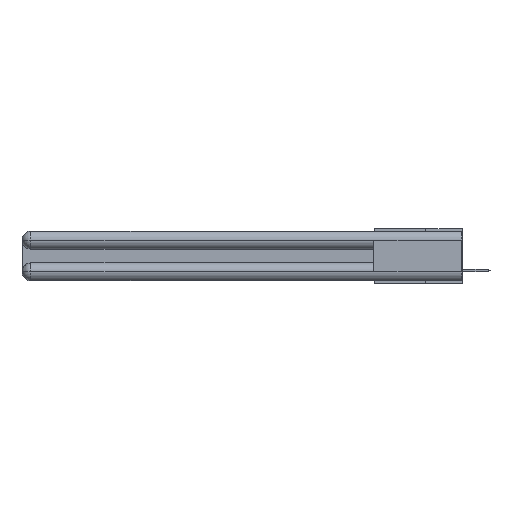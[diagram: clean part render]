
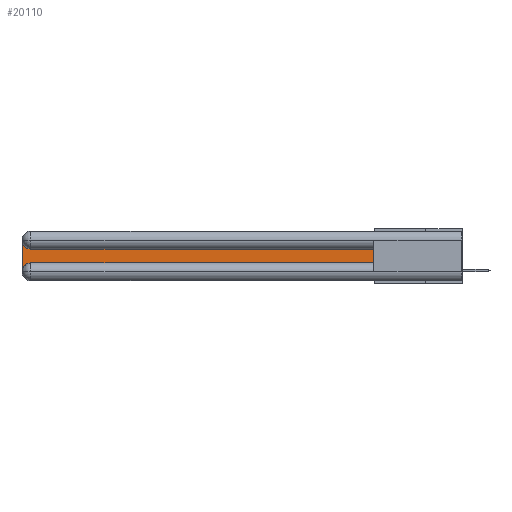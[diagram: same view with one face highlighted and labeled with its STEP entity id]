
A CAD part, left-side view. The second image highlights one B-rep face of the part: STEP entity #20110.
In plain terms, the highlighted planar face has unit normal (-1, 0, 0).
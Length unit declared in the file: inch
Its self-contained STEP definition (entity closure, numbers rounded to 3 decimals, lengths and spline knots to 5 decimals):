
#341 = EDGE_CURVE ( 'NONE', #3801, #3628, #25127, .T. ) ;
#884 = ORIENTED_EDGE ( 'NONE', *, *, #1741, .T. ) ;
#1289 = CARTESIAN_POINT ( 'NONE',  ( 0.075, 3., -0.0625 ) ) ;
#1308 = DIRECTION ( 'NONE',  ( 0., -1., 0. ) ) ;
#1741 = EDGE_CURVE ( 'NONE', #25825, #18079, #4606, .T. ) ;
#1869 = DIRECTION ( 'NONE',  ( 1., 0., 0. ) ) ;
#2002 = CARTESIAN_POINT ( 'NONE',  ( 0.075, 2.94, -0.1225 ) ) ;
#2137 = CARTESIAN_POINT ( 'NONE',  ( 0.075, 2.94, -0.0625 ) ) ;
#2150 = CARTESIAN_POINT ( 'NONE',  ( 0.075, 0.6, -0.1225 ) ) ;
#2297 = ORIENTED_EDGE ( 'NONE', *, *, #25579, .T. ) ;
#2655 = CARTESIAN_POINT ( 'NONE',  ( 0.075, 2.94, -0.2775 ) ) ;
#3628 = VERTEX_POINT ( 'NONE', #24005 ) ;
#3781 = DIRECTION ( 'NONE',  ( 0., 0., -1. ) ) ;
#3801 = VERTEX_POINT ( 'NONE', #18341 ) ;
#4606 = LINE ( 'NONE', #4968, #11680 ) ;
#4782 = DIRECTION ( 'NONE',  ( 0., 1., 0. ) ) ;
#4968 = CARTESIAN_POINT ( 'NONE',  ( 0.075, 0.6, -0.1225 ) ) ;
#5017 = LINE ( 'NONE', #17760, #25535 ) ;
#5760 = PLANE ( 'NONE',  #20091 ) ;
#5998 = DIRECTION ( 'NONE',  ( 1., 0., 0. ) ) ;
#6035 = FACE_OUTER_BOUND ( 'NONE', #15316, .T. ) ;
#6189 = EDGE_CURVE ( 'NONE', #3628, #25825, #5017, .T. ) ;
#6863 = VECTOR ( 'NONE', #1308, 39.37008 ) ;
#6967 = CARTESIAN_POINT ( 'NONE',  ( 0.075, 3., -0.2175 ) ) ;
#8753 = VERTEX_POINT ( 'NONE', #10257 ) ;
#9004 = ORIENTED_EDGE ( 'NONE', *, *, #16251, .T. ) ;
#10257 = CARTESIAN_POINT ( 'NONE',  ( 0.075, 3., -0.2775 ) ) ;
#10834 = DIRECTION ( 'NONE',  ( 0., 0., -1. ) ) ;
#11265 = DIRECTION ( 'NONE',  ( 0., 0., -1. ) ) ;
#11680 = VECTOR ( 'NONE', #4782, 39.37008 ) ;
#12953 = VERTEX_POINT ( 'NONE', #1289 ) ;
#15316 = EDGE_LOOP ( 'NONE', ( #884, #23331, #2297, #9004, #18621, #25317 ) ) ;
#16251 = EDGE_CURVE ( 'NONE', #8753, #3801, #23530, .T. ) ;
#16760 = EDGE_CURVE ( 'NONE', #18079, #12953, #17458, .T. ) ;
#17458 = CIRCLE ( 'NONE', #26164, 0.06 ) ;
#17607 = AXIS2_PLACEMENT_3D ( 'NONE', #2655, #5998, #11265 ) ;
#17760 = CARTESIAN_POINT ( 'NONE',  ( 0.075, 0.6, -0.2175 ) ) ;
#18079 = VERTEX_POINT ( 'NONE', #2002 ) ;
#18341 = CARTESIAN_POINT ( 'NONE',  ( 0.075, 2.94, -0.2175 ) ) ;
#18621 = ORIENTED_EDGE ( 'NONE', *, *, #341, .T. ) ;
#20091 = AXIS2_PLACEMENT_3D ( 'NONE', #22268, #1869, #3781 ) ;
#20110 = ADVANCED_FACE ( 'NONE', ( #6035 ), #5760, .F. ) ;
#20683 = DIRECTION ( 'NONE',  ( 1., 0., 0. ) ) ;
#21752 = VECTOR ( 'NONE', #10834, 39.37008 ) ;
#22268 = CARTESIAN_POINT ( 'NONE',  ( 0.075, 3., -0.1225 ) ) ;
#22802 = DIRECTION ( 'NONE',  ( 0., 0., -1. ) ) ;
#23331 = ORIENTED_EDGE ( 'NONE', *, *, #16760, .T. ) ;
#23530 = CIRCLE ( 'NONE', #17607, 0.06 ) ;
#23605 = DIRECTION ( 'NONE',  ( 0., 0., 1. ) ) ;
#23736 = CARTESIAN_POINT ( 'NONE',  ( 0.075, 0.6, -0.2175 ) ) ;
#24005 = CARTESIAN_POINT ( 'NONE',  ( 0.075, 0.6, -0.2175 ) ) ;
#24307 = LINE ( 'NONE', #6967, #21752 ) ;
#25127 = LINE ( 'NONE', #23736, #6863 ) ;
#25317 = ORIENTED_EDGE ( 'NONE', *, *, #6189, .T. ) ;
#25535 = VECTOR ( 'NONE', #23605, 39.37008 ) ;
#25579 = EDGE_CURVE ( 'NONE', #12953, #8753, #24307, .T. ) ;
#25825 = VERTEX_POINT ( 'NONE', #2150 ) ;
#26164 = AXIS2_PLACEMENT_3D ( 'NONE', #2137, #20683, #22802 ) ;
